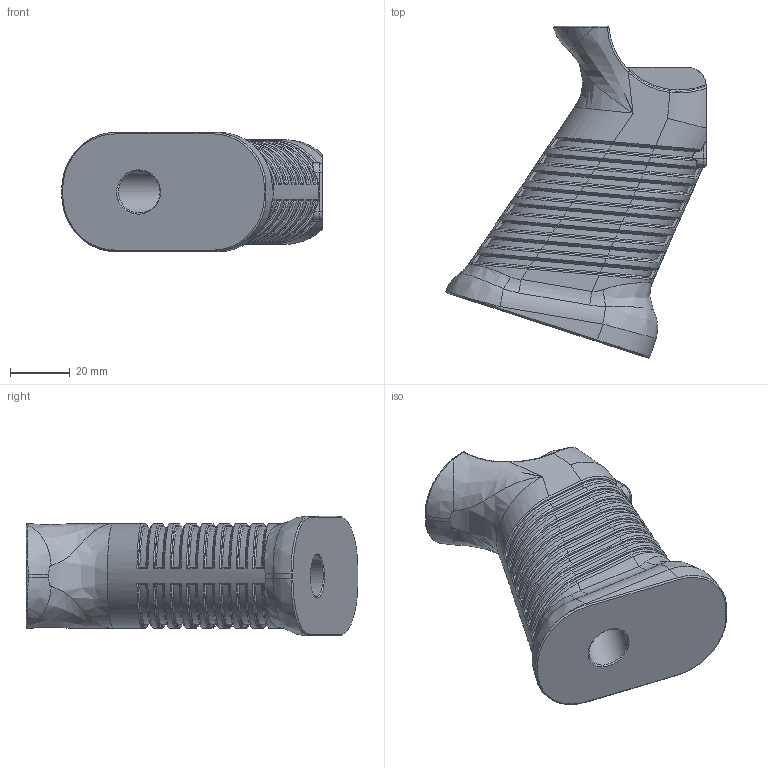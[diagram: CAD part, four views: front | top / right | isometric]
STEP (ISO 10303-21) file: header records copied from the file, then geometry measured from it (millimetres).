
FILE_DESCRIPTION (( 'STEP AP203' ), '1' );
FILE_NAME ('WTF-9_pistol_grip_fixed.STEP', '2020-05-13T07:59:37', ( '' ), ( '' ), 'SwSTEP 2.0', 'SolidWorks 2016', '' );
FILE_SCHEMA (( 'CONFIG_CONTROL_DESIGN' ));
Length unit declared in the file: millimetre
Products named in the file (1): WTF-9_pistol_grip_fixed
Bounding box: 87.31 x 111.25 x 40 mm (x, y, z)
Volume: 134835 mm3; surface area: 25696.1 mm2
Topology: 1 solids, 1 shells, 637 faces, 1727 edges, 1091 vertices
Faces by surface type: bspline 327, plane 220, cylinder 73, cone 9, torus 8
Full cylindrical faces by diameter (mm): 3.962 x1, 5.9 x1, 14 x1
Entity records: 32399 total; most frequent: CARTESIAN_POINT 18789, ORIENTED_EDGE 3424, DIRECTION 1760, EDGE_CURVE 1712, VERTEX_POINT 1086, VECTOR 894, LINE 894, EDGE_LOOP 648
